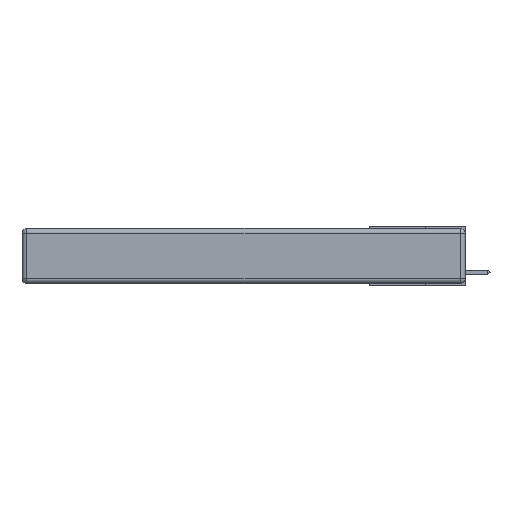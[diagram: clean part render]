
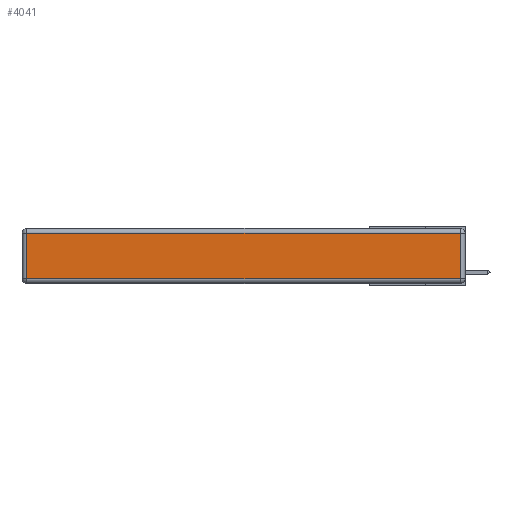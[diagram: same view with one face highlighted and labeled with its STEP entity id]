
A CAD part, left-side view. The second image highlights one B-rep face of the part: STEP entity #4041.
In plain terms, the highlighted planar face has unit normal (-1, 0, 0).
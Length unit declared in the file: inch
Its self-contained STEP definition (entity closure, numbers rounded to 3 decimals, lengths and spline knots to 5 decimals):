
#5 = VERTEX_POINT ( 'NONE', #7654 ) ;
#18 = CARTESIAN_POINT ( 'NONE',  ( 0., 2.75, -0.03 ) ) ;
#1310 = ORIENTED_EDGE ( 'NONE', *, *, #8198, .T. ) ;
#1653 = CARTESIAN_POINT ( 'NONE',  ( 0., 0., -0.313 ) ) ;
#2119 = CARTESIAN_POINT ( 'NONE',  ( 0., 2.72, -0.343 ) ) ;
#2222 = VERTEX_POINT ( 'NONE', #3740 ) ;
#2235 = EDGE_CURVE ( 'NONE', #2445, #5, #4167, .T. ) ;
#2378 = VERTEX_POINT ( 'NONE', #5416 ) ;
#2445 = VERTEX_POINT ( 'NONE', #8293 ) ;
#2645 = VECTOR ( 'NONE', #6686, 39.37008 ) ;
#2937 = LINE ( 'NONE', #12730, #2645 ) ;
#3121 = DIRECTION ( 'NONE',  ( 0., 0., -1. ) ) ;
#3740 = CARTESIAN_POINT ( 'NONE',  ( 0., 0.03, -0.03 ) ) ;
#4041 = ADVANCED_FACE ( 'NONE', ( #5843 ), #9445, .T. ) ;
#4167 = LINE ( 'NONE', #1653, #7680 ) ;
#5416 = CARTESIAN_POINT ( 'NONE',  ( 0., 2.72, -0.03 ) ) ;
#5843 = FACE_OUTER_BOUND ( 'NONE', #13068, .T. ) ;
#6298 = DIRECTION ( 'NONE',  ( -1., 0., 0. ) ) ;
#6415 = VECTOR ( 'NONE', #3121, 39.37008 ) ;
#6417 = ORIENTED_EDGE ( 'NONE', *, *, #9567, .T. ) ;
#6686 = DIRECTION ( 'NONE',  ( 0., 0., 1. ) ) ;
#6864 = ORIENTED_EDGE ( 'NONE', *, *, #2235, .T. ) ;
#7654 = CARTESIAN_POINT ( 'NONE',  ( 0., 0.03, -0.313 ) ) ;
#7680 = VECTOR ( 'NONE', #7759, 39.37008 ) ;
#7759 = DIRECTION ( 'NONE',  ( 0., -1., 0. ) ) ;
#8198 = EDGE_CURVE ( 'NONE', #2378, #2445, #11705, .T. ) ;
#8293 = CARTESIAN_POINT ( 'NONE',  ( 0., 2.72, -0.313 ) ) ;
#8356 = EDGE_CURVE ( 'NONE', #5, #2222, #2937, .T. ) ;
#8577 = ORIENTED_EDGE ( 'NONE', *, *, #8356, .T. ) ;
#8615 = VECTOR ( 'NONE', #12228, 39.37008 ) ;
#9231 = LINE ( 'NONE', #18, #8615 ) ;
#9357 = CARTESIAN_POINT ( 'NONE',  ( 0., 0., -0.343 ) ) ;
#9445 = PLANE ( 'NONE',  #9568 ) ;
#9567 = EDGE_CURVE ( 'NONE', #2222, #2378, #9231, .T. ) ;
#9568 = AXIS2_PLACEMENT_3D ( 'NONE', #9357, #6298, #12453 ) ;
#11705 = LINE ( 'NONE', #2119, #6415 ) ;
#12228 = DIRECTION ( 'NONE',  ( 0., 1., 0. ) ) ;
#12453 = DIRECTION ( 'NONE',  ( 0., 0., 1. ) ) ;
#12730 = CARTESIAN_POINT ( 'NONE',  ( 0., 0.03, -0.343 ) ) ;
#13068 = EDGE_LOOP ( 'NONE', ( #6864, #8577, #6417, #1310 ) ) ;
